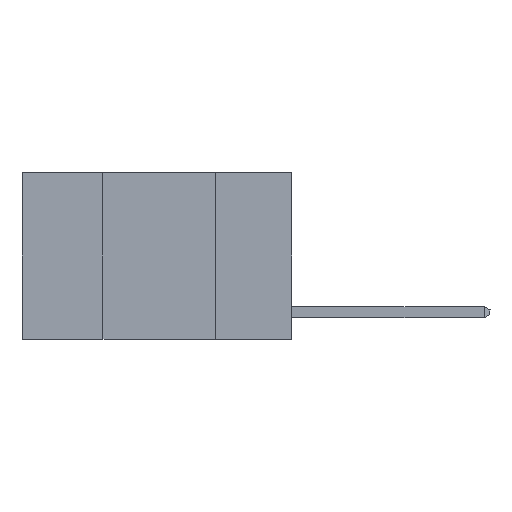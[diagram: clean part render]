
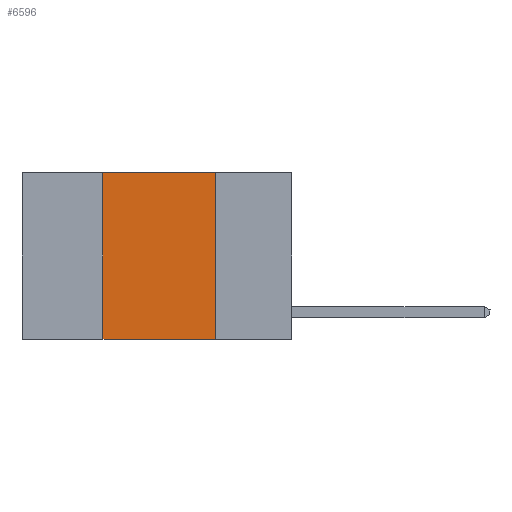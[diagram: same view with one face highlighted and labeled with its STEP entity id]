
A CAD part, left-side view. The second image highlights one B-rep face of the part: STEP entity #6596.
In plain terms, the highlighted planar face has unit normal (-1, 0, 0).
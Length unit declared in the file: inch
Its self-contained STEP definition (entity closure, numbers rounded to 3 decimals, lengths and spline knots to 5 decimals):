
#285 = DIRECTION ( 'NONE',  ( 1., 0., 0. ) ) ;
#330 = VERTEX_POINT ( 'NONE', #10705 ) ;
#453 = CARTESIAN_POINT ( 'NONE',  ( 0., 0.42, 0. ) ) ;
#1594 = EDGE_CURVE ( 'NONE', #8583, #2168, #6261, .T. ) ;
#1840 = CARTESIAN_POINT ( 'NONE',  ( 0., 0.42, 0. ) ) ;
#1847 = ORIENTED_EDGE ( 'NONE', *, *, #10800, .F. ) ;
#1904 = CARTESIAN_POINT ( 'NONE',  ( 0., 0.17, -0.37 ) ) ;
#2097 = LINE ( 'NONE', #1840, #5269 ) ;
#2168 = VERTEX_POINT ( 'NONE', #1904 ) ;
#2717 = LINE ( 'NONE', #5736, #11295 ) ;
#2992 = ORIENTED_EDGE ( 'NONE', *, *, #5787, .F. ) ;
#3025 = CARTESIAN_POINT ( 'NONE',  ( 0., 0.6, 0. ) ) ;
#3698 = FACE_OUTER_BOUND ( 'NONE', #10084, .T. ) ;
#4604 = DIRECTION ( 'NONE',  ( 0., -1., 0. ) ) ;
#5269 = VECTOR ( 'NONE', #11821, 39.37008 ) ;
#5348 = CARTESIAN_POINT ( 'NONE',  ( 0., 0.17, 0. ) ) ;
#5736 = CARTESIAN_POINT ( 'NONE',  ( 0., 0.6, 0. ) ) ;
#5787 = EDGE_CURVE ( 'NONE', #8583, #11703, #2097, .T. ) ;
#5960 = VECTOR ( 'NONE', #4604, 39.37008 ) ;
#6261 = LINE ( 'NONE', #9693, #5960 ) ;
#6596 = ADVANCED_FACE ( 'NONE', ( #3698 ), #7582, .F. ) ;
#6636 = DIRECTION ( 'NONE',  ( 0., -1., 0. ) ) ;
#6787 = DIRECTION ( 'NONE',  ( 0., 0., -1. ) ) ;
#7448 = ORIENTED_EDGE ( 'NONE', *, *, #1594, .T. ) ;
#7582 = PLANE ( 'NONE',  #10563 ) ;
#8583 = VERTEX_POINT ( 'NONE', #10346 ) ;
#9693 = CARTESIAN_POINT ( 'NONE',  ( 0., 0.6, -0.37 ) ) ;
#9835 = ORIENTED_EDGE ( 'NONE', *, *, #10358, .F. ) ;
#9906 = DIRECTION ( 'NONE',  ( 0., 0., -1. ) ) ;
#10084 = EDGE_LOOP ( 'NONE', ( #1847, #9835, #2992, #7448 ) ) ;
#10346 = CARTESIAN_POINT ( 'NONE',  ( 0., 0.42, -0.37 ) ) ;
#10358 = EDGE_CURVE ( 'NONE', #11703, #330, #2717, .T. ) ;
#10563 = AXIS2_PLACEMENT_3D ( 'NONE', #3025, #285, #6787 ) ;
#10705 = CARTESIAN_POINT ( 'NONE',  ( 0., 0.17, 0. ) ) ;
#10709 = VECTOR ( 'NONE', #9906, 39.37008 ) ;
#10800 = EDGE_CURVE ( 'NONE', #330, #2168, #11130, .T. ) ;
#11130 = LINE ( 'NONE', #5348, #10709 ) ;
#11295 = VECTOR ( 'NONE', #6636, 39.37008 ) ;
#11703 = VERTEX_POINT ( 'NONE', #453 ) ;
#11821 = DIRECTION ( 'NONE',  ( 0., 0., 1. ) ) ;
